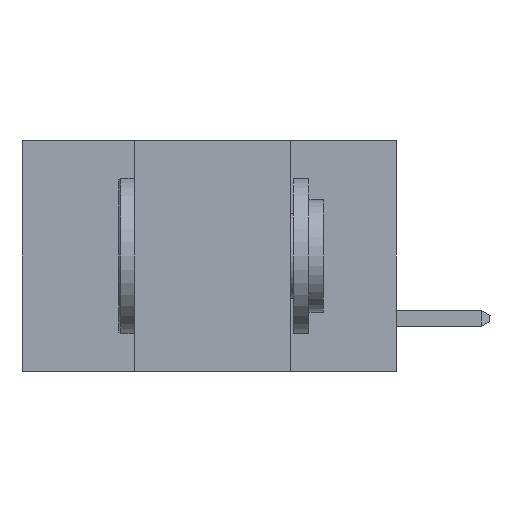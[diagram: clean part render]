
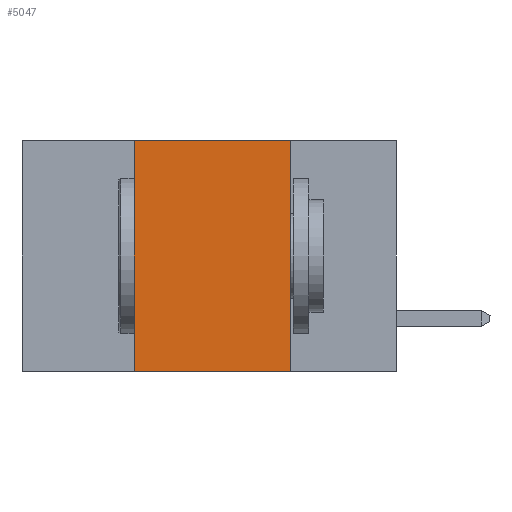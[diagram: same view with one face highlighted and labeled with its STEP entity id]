
A CAD part, left-side view. The second image highlights one B-rep face of the part: STEP entity #5047.
In plain terms, the highlighted planar face has unit normal (-1, 0, 0).
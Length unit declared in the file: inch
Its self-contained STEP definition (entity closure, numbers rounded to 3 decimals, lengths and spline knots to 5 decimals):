
#2013 = LINE ( 'NONE', #7156, #7760 ) ;
#2049 = CARTESIAN_POINT ( 'NONE',  ( 0., 0.42, -0.37 ) ) ;
#2145 = DIRECTION ( 'NONE',  ( 0., 0., -1. ) ) ;
#2176 = ORIENTED_EDGE ( 'NONE', *, *, #10673, .F. ) ;
#2252 = DIRECTION ( 'NONE',  ( 0., 0., 1. ) ) ;
#2992 = CARTESIAN_POINT ( 'NONE',  ( 0., 0.17, -0.37 ) ) ;
#3073 = EDGE_CURVE ( 'NONE', #3928, #9852, #2013, .T. ) ;
#3096 = EDGE_CURVE ( 'NONE', #9852, #9535, #12678, .T. ) ;
#3129 = DIRECTION ( 'NONE',  ( 1., 0., 0. ) ) ;
#3201 = PLANE ( 'NONE',  #11167 ) ;
#3279 = VECTOR ( 'NONE', #2145, 39.37008 ) ;
#3472 = DIRECTION ( 'NONE',  ( 0., -1., 0. ) ) ;
#3928 = VERTEX_POINT ( 'NONE', #4017 ) ;
#4017 = CARTESIAN_POINT ( 'NONE',  ( 0., 0.42, 0. ) ) ;
#4339 = CARTESIAN_POINT ( 'NONE',  ( 0., 0.42, -0.37 ) ) ;
#4941 = ORIENTED_EDGE ( 'NONE', *, *, #3096, .F. ) ;
#5047 = ADVANCED_FACE ( 'NONE', ( #12883 ), #3201, .F. ) ;
#5673 = VECTOR ( 'NONE', #3472, 39.37008 ) ;
#5680 = EDGE_LOOP ( 'NONE', ( #4941, #6667, #2176, #13361 ) ) ;
#6667 = ORIENTED_EDGE ( 'NONE', *, *, #3073, .F. ) ;
#7156 = CARTESIAN_POINT ( 'NONE',  ( 0., 0.6, 0. ) ) ;
#7431 = DIRECTION ( 'NONE',  ( 0., -1., 0. ) ) ;
#7760 = VECTOR ( 'NONE', #7431, 39.37008 ) ;
#8597 = LINE ( 'NONE', #2049, #12637 ) ;
#8747 = CARTESIAN_POINT ( 'NONE',  ( 0., 0.6, -0.37 ) ) ;
#9535 = VERTEX_POINT ( 'NONE', #11138 ) ;
#9852 = VERTEX_POINT ( 'NONE', #12691 ) ;
#10094 = LINE ( 'NONE', #8747, #5673 ) ;
#10673 = EDGE_CURVE ( 'NONE', #11591, #3928, #8597, .T. ) ;
#10818 = DIRECTION ( 'NONE',  ( 0., 0., -1. ) ) ;
#11138 = CARTESIAN_POINT ( 'NONE',  ( 0., 0.17, -0.37 ) ) ;
#11167 = AXIS2_PLACEMENT_3D ( 'NONE', #13023, #3129, #10818 ) ;
#11591 = VERTEX_POINT ( 'NONE', #4339 ) ;
#12637 = VECTOR ( 'NONE', #2252, 39.37008 ) ;
#12678 = LINE ( 'NONE', #2992, #3279 ) ;
#12691 = CARTESIAN_POINT ( 'NONE',  ( 0., 0.17, 0. ) ) ;
#12883 = FACE_OUTER_BOUND ( 'NONE', #5680, .T. ) ;
#13023 = CARTESIAN_POINT ( 'NONE',  ( 0., 0.6, 0. ) ) ;
#13292 = EDGE_CURVE ( 'NONE', #11591, #9535, #10094, .T. ) ;
#13361 = ORIENTED_EDGE ( 'NONE', *, *, #13292, .T. ) ;
